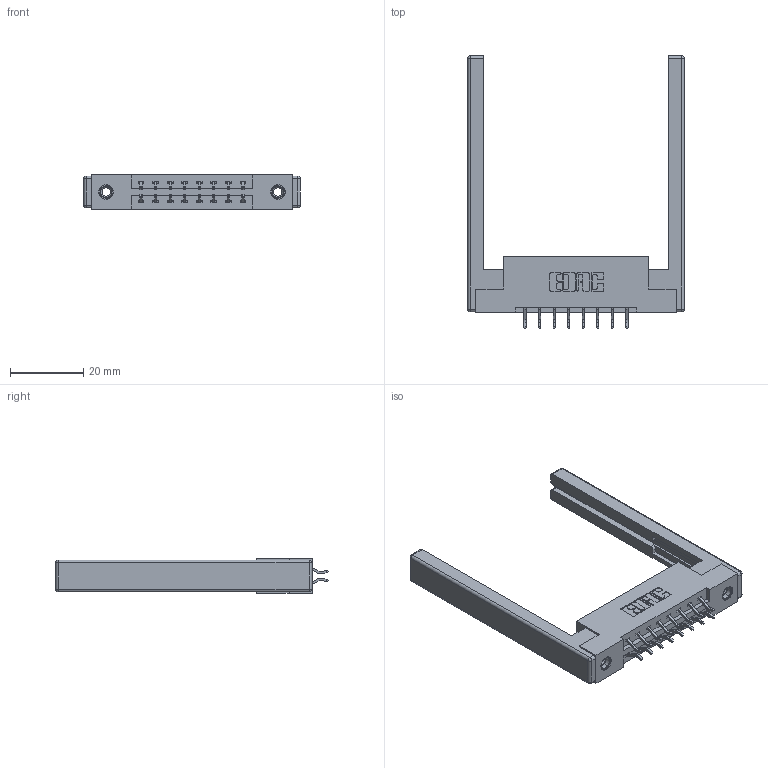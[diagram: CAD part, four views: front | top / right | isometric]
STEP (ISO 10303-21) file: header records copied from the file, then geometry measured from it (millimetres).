
FILE_DESCRIPTION (( 'STEP AP203' ), '1' );
FILE_NAME ('387-016-556-268.STEP', '2019-10-15T23:49:11', ( '' ), ( '' ), 'SwSTEP 2.0', 'SolidWorks 2016', '' );
FILE_SCHEMA (( 'CONFIG_CONTROL_DESIGN' ));
Length unit declared in the file: inch
Products named in the file (5): 307-220-068; 345-250-001_345-250-001-102; 387-016-556-268; 337 Part_Flush Mounting Lugs - 0.156 Dia-TI; 345-292-001_556 Tail
Assembly tree (21 placements, depth 2):
  387-016-556-268
    337 Part_Flush Mounting Lugs - 0.156 Dia-TI
    345-292-001_556 Tail  x16
    345-250-001_345-250-001-102  x2
    307-220-068  x2
Bounding box: 59.13 x 74.31 x 9.4 mm (x, y, z)
Volume: 10163.3 mm3; surface area: 10219.8 mm2
Topology: 21 solids, 21 shells, 1228 faces, 3565 edges, 2334 vertices
Faces by surface type: plane 830, cylinder 374, cone 12, sphere 8, torus 4
Entity records: 13580 total; most frequent: CARTESIAN_POINT 2295, ORIENTED_EDGE 2208, DIRECTION 2074, EDGE_CURVE 1104, LINE 918, VECTOR 918, VERTEX_POINT 726, AXIS2_PLACEMENT_3D 578
